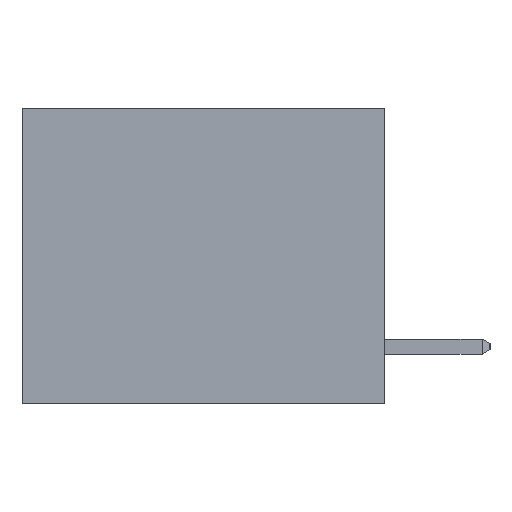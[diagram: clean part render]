
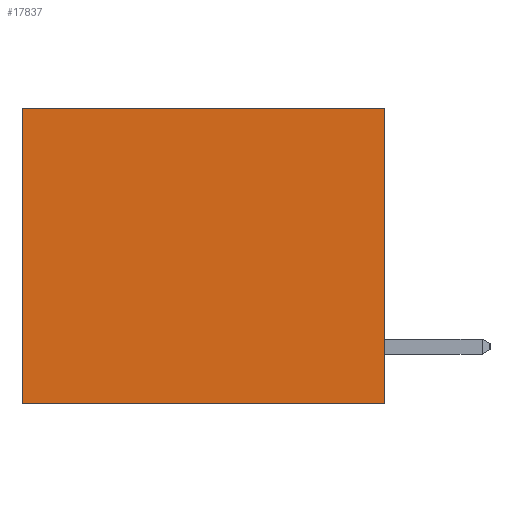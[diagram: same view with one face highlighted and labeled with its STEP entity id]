
A CAD part, left-side view. The second image highlights one B-rep face of the part: STEP entity #17837.
In plain terms, the highlighted planar face has unit normal (-1, 0, 0).
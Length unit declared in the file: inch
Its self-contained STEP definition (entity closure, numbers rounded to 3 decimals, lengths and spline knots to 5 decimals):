
#306 = VERTEX_POINT ( 'NONE', #4187 ) ;
#2240 = VERTEX_POINT ( 'NONE', #4958 ) ;
#2274 = DIRECTION ( 'NONE',  ( 0., 0., -1. ) ) ;
#2745 = CARTESIAN_POINT ( 'NONE',  ( 0.3165, 0., -0.49 ) ) ;
#4187 = CARTESIAN_POINT ( 'NONE',  ( 0.3165, 0., 0. ) ) ;
#4744 = EDGE_LOOP ( 'NONE', ( #22974, #18104, #8038, #17407 ) ) ;
#4761 = LINE ( 'NONE', #6991, #14244 ) ;
#4958 = CARTESIAN_POINT ( 'NONE',  ( 0.3165, 0.6, -0.49 ) ) ;
#5417 = DIRECTION ( 'NONE',  ( 0., 0., -1. ) ) ;
#5530 = LINE ( 'NONE', #10719, #22178 ) ;
#5803 = VECTOR ( 'NONE', #16558, 39.37008 ) ;
#6966 = CARTESIAN_POINT ( 'NONE',  ( 0.3165, 0., -0.49 ) ) ;
#6980 = LINE ( 'NONE', #2745, #18951 ) ;
#6991 = CARTESIAN_POINT ( 'NONE',  ( 0.3165, 0., 0. ) ) ;
#7136 = DIRECTION ( 'NONE',  ( 1., 0., 0. ) ) ;
#7157 = DIRECTION ( 'NONE',  ( 0., 1., 0. ) ) ;
#7970 = CARTESIAN_POINT ( 'NONE',  ( 0.3165, 0.6, 0. ) ) ;
#8038 = ORIENTED_EDGE ( 'NONE', *, *, #20870, .F. ) ;
#8755 = CARTESIAN_POINT ( 'NONE',  ( 0.3165, 0., -0.49 ) ) ;
#9292 = EDGE_CURVE ( 'NONE', #306, #14547, #4761, .T. ) ;
#10156 = VERTEX_POINT ( 'NONE', #6966 ) ;
#10447 = EDGE_CURVE ( 'NONE', #10156, #2240, #16383, .T. ) ;
#10719 = CARTESIAN_POINT ( 'NONE',  ( 0.3165, 0.6, -0.49 ) ) ;
#12295 = CARTESIAN_POINT ( 'NONE',  ( 0.3165, 0., -0.49 ) ) ;
#13003 = EDGE_CURVE ( 'NONE', #14547, #2240, #5530, .T. ) ;
#14244 = VECTOR ( 'NONE', #7157, 39.37008 ) ;
#14547 = VERTEX_POINT ( 'NONE', #7970 ) ;
#15698 = DIRECTION ( 'NONE',  ( 0., 0., -1. ) ) ;
#16383 = LINE ( 'NONE', #12295, #5803 ) ;
#16558 = DIRECTION ( 'NONE',  ( 0., 1., 0. ) ) ;
#17368 = FACE_OUTER_BOUND ( 'NONE', #4744, .T. ) ;
#17407 = ORIENTED_EDGE ( 'NONE', *, *, #9292, .T. ) ;
#17837 = ADVANCED_FACE ( 'NONE', ( #17368 ), #18757, .F. ) ;
#18005 = AXIS2_PLACEMENT_3D ( 'NONE', #8755, #7136, #15698 ) ;
#18104 = ORIENTED_EDGE ( 'NONE', *, *, #10447, .F. ) ;
#18757 = PLANE ( 'NONE',  #18005 ) ;
#18951 = VECTOR ( 'NONE', #2274, 39.37008 ) ;
#20870 = EDGE_CURVE ( 'NONE', #306, #10156, #6980, .T. ) ;
#22178 = VECTOR ( 'NONE', #5417, 39.37008 ) ;
#22974 = ORIENTED_EDGE ( 'NONE', *, *, #13003, .T. ) ;
